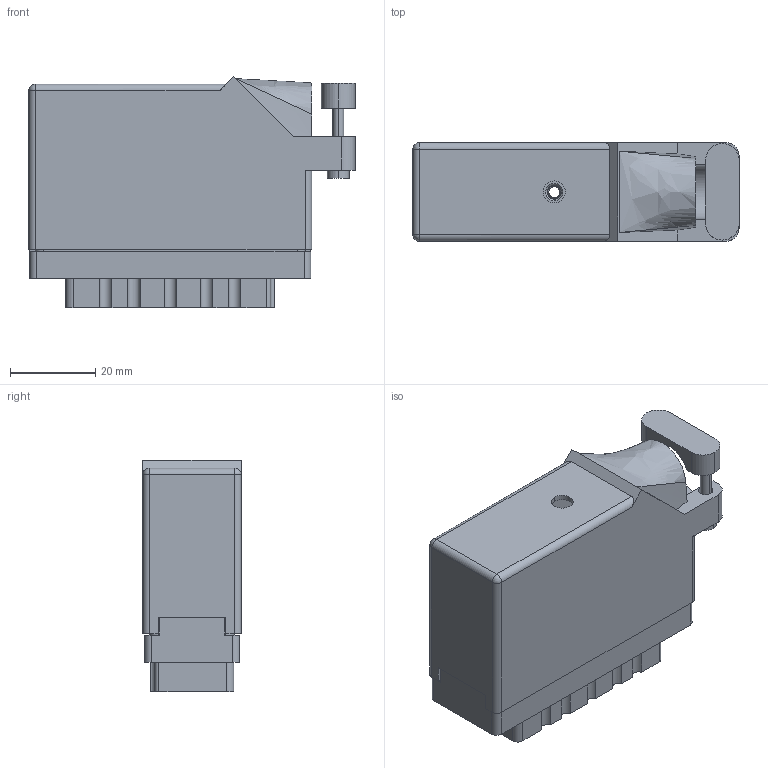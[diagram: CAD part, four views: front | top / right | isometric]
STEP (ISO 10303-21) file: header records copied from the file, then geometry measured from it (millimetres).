
FILE_DESCRIPTION (( 'STEP AP203' ), '1' );
FILE_NAME ('516-056-000-626.STEP', '2020-03-05T20:40:32', ( '' ), ( '' ), 'SwSTEP 2.0', 'SolidWorks 2016', '' );
FILE_SCHEMA (( 'CONFIG_CONTROL_DESIGN' ));
Length unit declared in the file: inch
Products named in the file (4): 516-252-035-100_516-252-035-100; 516-056-000-626; 516-230-001_Plastic - 056 Side Entry; 516 Part Receptacle_056
Assembly tree (3 placements, depth 2):
  516-056-000-626
    516 Part Receptacle_056
    516-230-001_Plastic - 056 Side Entry
    516-252-035-100_516-252-035-100
Bounding box: 76.5 x 23.11 x 54.15 mm (x, y, z)
Volume: 26643.1 mm3; surface area: 37216.6 mm2
Topology: 3 solids, 3 shells, 1390 faces, 4066 edges, 2704 vertices
Faces by surface type: plane 941, cylinder 426, cone 12, bspline 9, sphere 2
Entity records: 49157 total; most frequent: CARTESIAN_POINT 10703, ORIENTED_EDGE 8128, DIRECTION 7847, EDGE_CURVE 4064, VECTOR 2947, LINE 2947, VERTEX_POINT 2704, AXIS2_PLACEMENT_3D 2450
